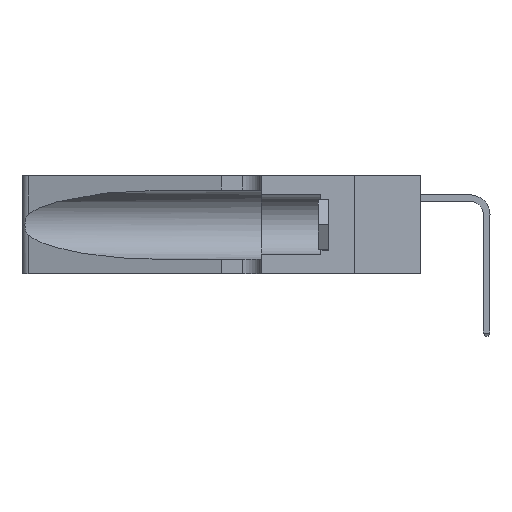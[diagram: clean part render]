
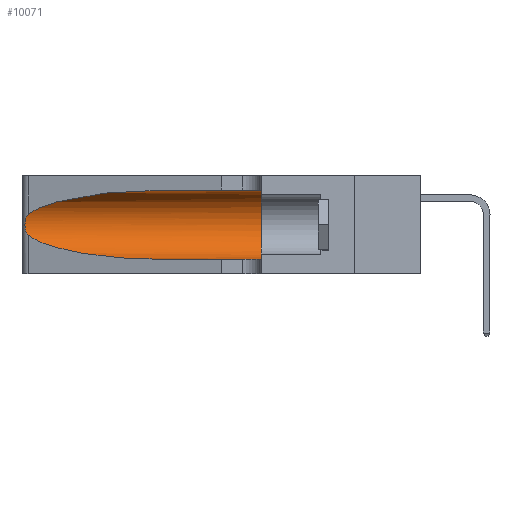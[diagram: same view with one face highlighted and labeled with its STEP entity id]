
A CAD part, left-side view. The second image highlights one B-rep face of the part: STEP entity #10071.
In plain terms, the highlighted cylindrical face has radius 3.308 mm (diameter 6.617 mm), a partial arc.
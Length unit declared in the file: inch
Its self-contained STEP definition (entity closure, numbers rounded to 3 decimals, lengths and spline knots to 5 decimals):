
#1560 = CARTESIAN_POINT ( 'NONE',  ( 0.1305, 0.72297, 0.31525 ) ) ;
#1573 = ORIENTED_EDGE ( 'NONE', *, *, #5270, .T. ) ;
#1728 = CARTESIAN_POINT ( 'NONE',  ( 0.25789, 1.23486, 0.15765 ) ) ;
#2024 = DIRECTION ( 'NONE',  ( 0., -1., 0. ) ) ;
#2075 = EDGE_CURVE ( 'NONE', #28246, #37390, #15302, .T. ) ;
#2763 = CARTESIAN_POINT ( 'NONE',  ( 0.1305, 0.35, 0.185 ) ) ;
#2982 = CARTESIAN_POINT ( 'NONE',  ( 0.25487, 1.22718, 0.14631 ) ) ;
#3102 = CARTESIAN_POINT ( 'NONE',  ( 0.1305, 0.72297, 0.05475 ) ) ;
#3780 = VERTEX_POINT ( 'NONE', #21027 ) ;
#4275 = DIRECTION ( 'NONE',  ( 0., 0., -1. ) ) ;
#4477 = ORIENTED_EDGE ( 'NONE', *, *, #11166, .T. ) ;
#4493 = CARTESIAN_POINT ( 'NONE',  ( 0.18966, 0.96281, 0.31525 ) ) ;
#4662 = CARTESIAN_POINT ( 'NONE',  ( 0.25555, 1.22993, 0.14849 ) ) ;
#5270 = EDGE_CURVE ( 'NONE', #3780, #19368, #5789, .T. ) ;
#5695 = DIRECTION ( 'NONE',  ( 0., 0., 1. ) ) ;
#5789 = LINE ( 'NONE', #22348, #12608 ) ;
#6158 = CARTESIAN_POINT ( 'NONE',  ( 0.1305, 0.35, 0.31525 ) ) ;
#6803 = AXIS2_PLACEMENT_3D ( 'NONE', #2763, #23055, #5695 ) ;
#7100 = CARTESIAN_POINT ( 'NONE',  ( 0.25487, 1.22718, 0.22369 ) ) ;
#7442 = CARTESIAN_POINT ( 'NONE',  ( 0.25487, 1.22718, 0.22369 ) ) ;
#7480 = CARTESIAN_POINT ( 'NONE',  ( 0.25639, 1.23184, 0.21858 ) ) ;
#7541 =( BOUNDED_CURVE ( )  B_SPLINE_CURVE ( 3, ( #2982, #34883, #20502, #3102 ),
 .UNSPECIFIED., .F., .F. ) 
 B_SPLINE_CURVE_WITH_KNOTS ( ( 4, 4 ),
 ( 3.44316, 4.71239 ),
 .UNSPECIFIED. ) 
 CURVE ( )  GEOMETRIC_REPRESENTATION_ITEM ( )  RATIONAL_B_SPLINE_CURVE ( ( 1., 0.87, 0.87, 1. ) ) 
 REPRESENTATION_ITEM ( '' )  );
#8716 = VERTEX_POINT ( 'NONE', #29566 ) ;
#9835 = ORIENTED_EDGE ( 'NONE', *, *, #2075, .T. ) ;
#10071 = ADVANCED_FACE ( 'NONE', ( #17066 ), #28771, .F. ) ;
#10392 = CARTESIAN_POINT ( 'NONE',  ( 0.25787, 1.23484, 0.2124 ) ) ;
#11166 = EDGE_CURVE ( 'NONE', #37390, #3780, #7541, .T. ) ;
#11409 = AXIS2_PLACEMENT_3D ( 'NONE', #21521, #36053, #4275 ) ;
#12608 = VECTOR ( 'NONE', #2024, 39.37008 ) ;
#13317 = CARTESIAN_POINT ( 'NONE',  ( 0.26018, 1.23835, 0.19895 ) ) ;
#13549 = VERTEX_POINT ( 'NONE', #6158 ) ;
#13836 = EDGE_CURVE ( 'NONE', #8716, #28246, #14270, .T. ) ;
#14270 =( BOUNDED_CURVE ( )  B_SPLINE_CURVE ( 3, ( #1560, #4493, #24754, #7442 ),
 .UNSPECIFIED., .F., .T. ) 
 B_SPLINE_CURVE_WITH_KNOTS ( ( 4, 4 ),
 ( 1.5708, 2.84003 ),
 .UNSPECIFIED. ) 
 CURVE ( )  GEOMETRIC_REPRESENTATION_ITEM ( )  RATIONAL_B_SPLINE_CURVE ( ( 1., 0.87, 0.87, 1. ) ) 
 REPRESENTATION_ITEM ( '' )  );
#14383 = VECTOR ( 'NONE', #23565, 39.37008 ) ;
#14404 = EDGE_LOOP ( 'NONE', ( #35144, #9835, #4477, #1573, #31664, #24365 ) ) ;
#14944 = CARTESIAN_POINT ( 'NONE',  ( 0.1305, 0.35, 0.05475 ) ) ;
#15302 = B_SPLINE_CURVE_WITH_KNOTS ( 'NONE', 3,
 ( #33432, #24802, #7480, #10392, #30638, #13317, #33547, #16269, #36433, #19151, #1728, #22046, #4662, #24919 ),
 .UNSPECIFIED., .F., .F.,
 ( 4, 2, 2, 2, 2, 2, 4 ),
 ( 0., 0.00027, 0.00053, 0.00107, 0.0016, 0.00187, 0.00214 ),
 .UNSPECIFIED. ) ;
#16269 = CARTESIAN_POINT ( 'NONE',  ( 0.26075, 1.23896, 0.178 ) ) ;
#17066 = FACE_OUTER_BOUND ( 'NONE', #14404, .T. ) ;
#19151 = CARTESIAN_POINT ( 'NONE',  ( 0.25856, 1.23593, 0.16098 ) ) ;
#19368 = VERTEX_POINT ( 'NONE', #14944 ) ;
#20502 = CARTESIAN_POINT ( 'NONE',  ( 0.18966, 0.96281, 0.05475 ) ) ;
#21027 = CARTESIAN_POINT ( 'NONE',  ( 0.1305, 0.72297, 0.05475 ) ) ;
#21521 = CARTESIAN_POINT ( 'NONE',  ( 0.1305, 1.61858, 0.185 ) ) ;
#22046 = CARTESIAN_POINT ( 'NONE',  ( 0.25639, 1.23186, 0.15144 ) ) ;
#22089 = LINE ( 'NONE', #35069, #14383 ) ;
#22348 = CARTESIAN_POINT ( 'NONE',  ( 0.1305, 1.61858, 0.05475 ) ) ;
#23055 = DIRECTION ( 'NONE',  ( 0., 1., 0. ) ) ;
#23565 = DIRECTION ( 'NONE',  ( 0., -1., 0. ) ) ;
#24365 = ORIENTED_EDGE ( 'NONE', *, *, #30734, .F. ) ;
#24754 = CARTESIAN_POINT ( 'NONE',  ( 0.2373, 1.15595, 0.28018 ) ) ;
#24802 = CARTESIAN_POINT ( 'NONE',  ( 0.25555, 1.22994, 0.2215 ) ) ;
#24919 = CARTESIAN_POINT ( 'NONE',  ( 0.25487, 1.22718, 0.14631 ) ) ;
#28246 = VERTEX_POINT ( 'NONE', #7100 ) ;
#28771 = CYLINDRICAL_SURFACE ( 'NONE', #11409, 0.13025 ) ;
#29566 = CARTESIAN_POINT ( 'NONE',  ( 0.1305, 0.72297, 0.31525 ) ) ;
#30638 = CARTESIAN_POINT ( 'NONE',  ( 0.25854, 1.2359, 0.20912 ) ) ;
#30734 = EDGE_CURVE ( 'NONE', #8716, #13549, #22089, .T. ) ;
#31664 = ORIENTED_EDGE ( 'NONE', *, *, #37474, .F. ) ;
#31684 = CIRCLE ( 'NONE', #6803, 0.13025 ) ;
#33432 = CARTESIAN_POINT ( 'NONE',  ( 0.25487, 1.22718, 0.22369 ) ) ;
#33547 = CARTESIAN_POINT ( 'NONE',  ( 0.26075, 1.23896, 0.19203 ) ) ;
#34073 = CARTESIAN_POINT ( 'NONE',  ( 0.25487, 1.22718, 0.14631 ) ) ;
#34883 = CARTESIAN_POINT ( 'NONE',  ( 0.2373, 1.15595, 0.08982 ) ) ;
#35069 = CARTESIAN_POINT ( 'NONE',  ( 0.1305, 1.61858, 0.31525 ) ) ;
#35144 = ORIENTED_EDGE ( 'NONE', *, *, #13836, .T. ) ;
#36053 = DIRECTION ( 'NONE',  ( 0., -1., 0. ) ) ;
#36433 = CARTESIAN_POINT ( 'NONE',  ( 0.26017, 1.23833, 0.17102 ) ) ;
#37390 = VERTEX_POINT ( 'NONE', #34073 ) ;
#37474 = EDGE_CURVE ( 'NONE', #13549, #19368, #31684, .T. ) ;
